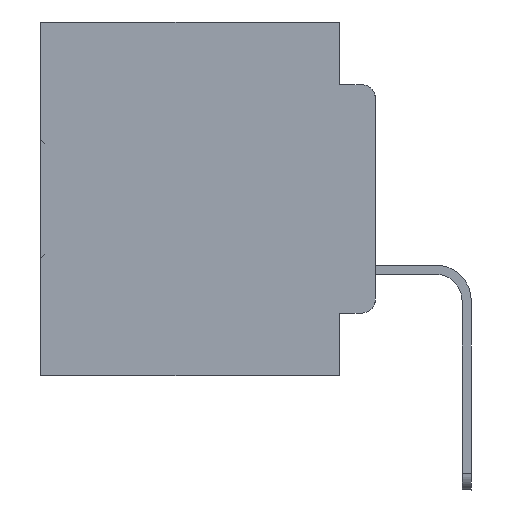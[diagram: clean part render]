
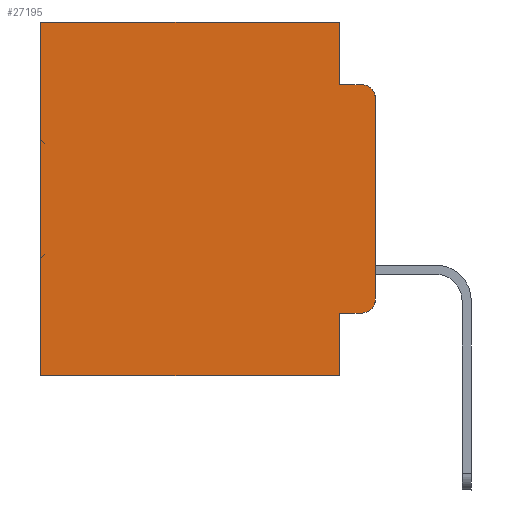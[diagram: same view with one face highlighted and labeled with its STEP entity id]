
A CAD part, left-side view. The second image highlights one B-rep face of the part: STEP entity #27195.
In plain terms, the highlighted planar face has unit normal (-1, 0, 0).
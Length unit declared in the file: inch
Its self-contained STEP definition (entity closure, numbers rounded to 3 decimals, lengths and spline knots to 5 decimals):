
#61 = VECTOR ( 'NONE', #29851, 39.37008 ) ;
#204 = LINE ( 'NONE', #7187, #8921 ) ;
#933 = VERTEX_POINT ( 'NONE', #10230 ) ;
#1137 = CARTESIAN_POINT ( 'NONE',  ( 0.298, 0.473, -0.5 ) ) ;
#1516 = VECTOR ( 'NONE', #14878, 39.37008 ) ;
#2811 = CARTESIAN_POINT ( 'NONE',  ( 0.298, 0., -0.3915 ) ) ;
#2867 = ORIENTED_EDGE ( 'NONE', *, *, #7134, .F. ) ;
#3169 = CARTESIAN_POINT ( 'NONE',  ( 0.298, 0., 0. ) ) ;
#3488 = EDGE_CURVE ( 'NONE', #4897, #7586, #21159, .T. ) ;
#3685 = LINE ( 'NONE', #21090, #4135 ) ;
#3699 = VECTOR ( 'NONE', #27476, 39.37008 ) ;
#3808 = ORIENTED_EDGE ( 'NONE', *, *, #3488, .F. ) ;
#4135 = VECTOR ( 'NONE', #13466, 39.37008 ) ;
#4136 = CARTESIAN_POINT ( 'NONE',  ( 0.298, 0.051, -0.5 ) ) ;
#4635 = EDGE_CURVE ( 'NONE', #933, #7470, #9510, .T. ) ;
#4654 = CARTESIAN_POINT ( 'NONE',  ( 0.298, 0.02, -0.1085 ) ) ;
#4897 = VERTEX_POINT ( 'NONE', #5207 ) ;
#5207 = CARTESIAN_POINT ( 'NONE',  ( 0.298, 0.051, -0.0885 ) ) ;
#5997 = ORIENTED_EDGE ( 'NONE', *, *, #7194, .F. ) ;
#6503 = DIRECTION ( 'NONE',  ( 0., 1., 0. ) ) ;
#6751 = CARTESIAN_POINT ( 'NONE',  ( 0.298, 0.051, -0.4115 ) ) ;
#6919 = PLANE ( 'NONE',  #27807 ) ;
#7134 = EDGE_CURVE ( 'NONE', #18311, #27917, #3685, .T. ) ;
#7187 = CARTESIAN_POINT ( 'NONE',  ( 0.298, 0.473, 0. ) ) ;
#7194 = EDGE_CURVE ( 'NONE', #34146, #28284, #23547, .T. ) ;
#7259 = ORIENTED_EDGE ( 'NONE', *, *, #12107, .T. ) ;
#7470 = VERTEX_POINT ( 'NONE', #12068 ) ;
#7586 = VERTEX_POINT ( 'NONE', #31534 ) ;
#8921 = VECTOR ( 'NONE', #26063, 39.37008 ) ;
#8950 = AXIS2_PLACEMENT_3D ( 'NONE', #33889, #28983, #12993 ) ;
#9510 = LINE ( 'NONE', #33138, #10336 ) ;
#10230 = CARTESIAN_POINT ( 'NONE',  ( 0.298, 0.051, 0. ) ) ;
#10336 = VECTOR ( 'NONE', #6503, 39.37008 ) ;
#11415 = ORIENTED_EDGE ( 'NONE', *, *, #17761, .T. ) ;
#11517 = LINE ( 'NONE', #20597, #17724 ) ;
#11831 = EDGE_LOOP ( 'NONE', ( #5997, #11415, #3808, #26961, #16996, #14419, #19026, #2867, #7259, #18412 ) ) ;
#12068 = CARTESIAN_POINT ( 'NONE',  ( 0.298, 0.473, 0. ) ) ;
#12107 = EDGE_CURVE ( 'NONE', #18311, #28416, #16536, .T. ) ;
#12404 = EDGE_CURVE ( 'NONE', #933, #4897, #11517, .T. ) ;
#12993 = DIRECTION ( 'NONE',  ( 0., 0., -1. ) ) ;
#13466 = DIRECTION ( 'NONE',  ( 0., 0., -1. ) ) ;
#13913 = CARTESIAN_POINT ( 'NONE',  ( 0.298, 0.02, -0.4115 ) ) ;
#14419 = ORIENTED_EDGE ( 'NONE', *, *, #26622, .T. ) ;
#14878 = DIRECTION ( 'NONE',  ( 0., 1., 0. ) ) ;
#14891 = DIRECTION ( 'NONE',  ( 0., 0., -1. ) ) ;
#15162 = DIRECTION ( 'NONE',  ( 0., 0., -1. ) ) ;
#16523 = VECTOR ( 'NONE', #18884, 39.37008 ) ;
#16536 = LINE ( 'NONE', #6751, #3699 ) ;
#16996 = ORIENTED_EDGE ( 'NONE', *, *, #4635, .T. ) ;
#17205 = EDGE_CURVE ( 'NONE', #28416, #28284, #21521, .T. ) ;
#17427 = CARTESIAN_POINT ( 'NONE',  ( 0.298, 0.051, -0.4115 ) ) ;
#17724 = VECTOR ( 'NONE', #34089, 39.37008 ) ;
#17761 = EDGE_CURVE ( 'NONE', #34146, #7586, #29054, .T. ) ;
#18311 = VERTEX_POINT ( 'NONE', #17427 ) ;
#18412 = ORIENTED_EDGE ( 'NONE', *, *, #17205, .T. ) ;
#18884 = DIRECTION ( 'NONE',  ( 0., 0., -1. ) ) ;
#19026 = ORIENTED_EDGE ( 'NONE', *, *, #20100, .F. ) ;
#20100 = EDGE_CURVE ( 'NONE', #27917, #27057, #28463, .T. ) ;
#20597 = CARTESIAN_POINT ( 'NONE',  ( 0.298, 0.051, 0. ) ) ;
#21090 = CARTESIAN_POINT ( 'NONE',  ( 0.298, 0.051, 0. ) ) ;
#21159 = LINE ( 'NONE', #24377, #61 ) ;
#21521 = CIRCLE ( 'NONE', #8950, 0.02 ) ;
#23030 = DIRECTION ( 'NONE',  ( -1., 0., 0. ) ) ;
#23547 = LINE ( 'NONE', #3169, #16523 ) ;
#24219 = FACE_OUTER_BOUND ( 'NONE', #11831, .T. ) ;
#24377 = CARTESIAN_POINT ( 'NONE',  ( 0.298, 0.051, -0.0885 ) ) ;
#25455 = CARTESIAN_POINT ( 'NONE',  ( 0.298, 0., 0. ) ) ;
#26063 = DIRECTION ( 'NONE',  ( 0., 0., -1. ) ) ;
#26622 = EDGE_CURVE ( 'NONE', #7470, #27057, #204, .T. ) ;
#26961 = ORIENTED_EDGE ( 'NONE', *, *, #12404, .F. ) ;
#27057 = VERTEX_POINT ( 'NONE', #1137 ) ;
#27195 = ADVANCED_FACE ( 'NONE', ( #24219 ), #6919, .F. ) ;
#27476 = DIRECTION ( 'NONE',  ( 0., -1., 0. ) ) ;
#27807 = AXIS2_PLACEMENT_3D ( 'NONE', #25455, #30774, #14891 ) ;
#27917 = VERTEX_POINT ( 'NONE', #4136 ) ;
#28284 = VERTEX_POINT ( 'NONE', #2811 ) ;
#28416 = VERTEX_POINT ( 'NONE', #13913 ) ;
#28463 = LINE ( 'NONE', #33916, #1516 ) ;
#28983 = DIRECTION ( 'NONE',  ( -1., 0., 0. ) ) ;
#29054 = CIRCLE ( 'NONE', #33825, 0.02 ) ;
#29851 = DIRECTION ( 'NONE',  ( 0., -1., 0. ) ) ;
#30774 = DIRECTION ( 'NONE',  ( 1., 0., 0. ) ) ;
#30993 = CARTESIAN_POINT ( 'NONE',  ( 0.298, 0., -0.1085 ) ) ;
#31534 = CARTESIAN_POINT ( 'NONE',  ( 0.298, 0.02, -0.0885 ) ) ;
#33138 = CARTESIAN_POINT ( 'NONE',  ( 0.298, 0., 0. ) ) ;
#33825 = AXIS2_PLACEMENT_3D ( 'NONE', #4654, #23030, #15162 ) ;
#33889 = CARTESIAN_POINT ( 'NONE',  ( 0.298, 0.02, -0.3915 ) ) ;
#33916 = CARTESIAN_POINT ( 'NONE',  ( 0.298, 0., -0.5 ) ) ;
#34089 = DIRECTION ( 'NONE',  ( 0., 0., -1. ) ) ;
#34146 = VERTEX_POINT ( 'NONE', #30993 ) ;
